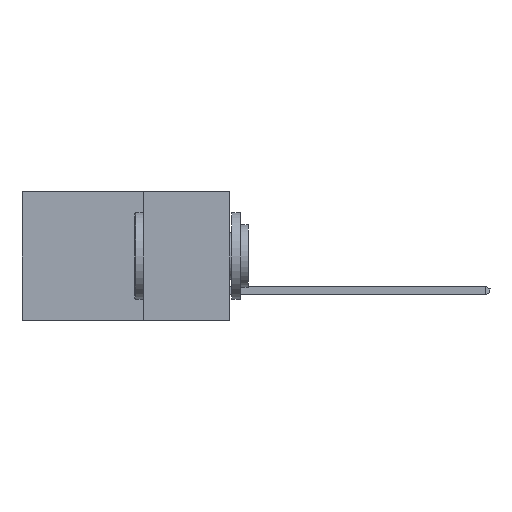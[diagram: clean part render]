
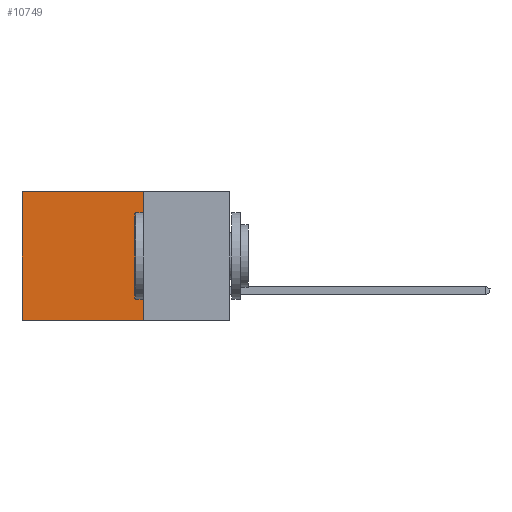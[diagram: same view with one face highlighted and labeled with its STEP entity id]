
A CAD part, left-side view. The second image highlights one B-rep face of the part: STEP entity #10749.
In plain terms, the highlighted planar face has unit normal (-1, 0, 0).
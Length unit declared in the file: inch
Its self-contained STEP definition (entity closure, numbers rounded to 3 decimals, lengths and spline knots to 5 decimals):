
#174 = ORIENTED_EDGE ( 'NONE', *, *, #14636, .F. ) ;
#426 = ORIENTED_EDGE ( 'NONE', *, *, #14293, .F. ) ;
#1193 = CARTESIAN_POINT ( 'NONE',  ( 0.2615, 0.25, -0.37 ) ) ;
#1228 = LINE ( 'NONE', #2352, #8386 ) ;
#1419 = CARTESIAN_POINT ( 'NONE',  ( 0.2615, 0.25, -0.37 ) ) ;
#2322 = LINE ( 'NONE', #1193, #9611 ) ;
#2352 = CARTESIAN_POINT ( 'NONE',  ( 0.2615, 0.6, -0.37 ) ) ;
#2372 = DIRECTION ( 'NONE',  ( 1., 0., 0. ) ) ;
#2518 = FACE_OUTER_BOUND ( 'NONE', #10405, .T. ) ;
#2593 = CARTESIAN_POINT ( 'NONE',  ( 0.2615, 0.25, 0. ) ) ;
#3091 = VERTEX_POINT ( 'NONE', #1419 ) ;
#3502 = PLANE ( 'NONE',  #11160 ) ;
#3981 = ORIENTED_EDGE ( 'NONE', *, *, #9873, .T. ) ;
#4097 = VERTEX_POINT ( 'NONE', #6072 ) ;
#4595 = CARTESIAN_POINT ( 'NONE',  ( 0.2615, 0.6, -0.37 ) ) ;
#5292 = LINE ( 'NONE', #7529, #10825 ) ;
#5918 = CARTESIAN_POINT ( 'NONE',  ( 0.2615, 0.25, 0. ) ) ;
#6072 = CARTESIAN_POINT ( 'NONE',  ( 0.2615, 0.6, 0. ) ) ;
#6815 = DIRECTION ( 'NONE',  ( 0., 1., 0. ) ) ;
#7054 = VERTEX_POINT ( 'NONE', #4595 ) ;
#7094 = CARTESIAN_POINT ( 'NONE',  ( 0.2615, 0.25, -0.37 ) ) ;
#7529 = CARTESIAN_POINT ( 'NONE',  ( 0.2615, 0.25, -0.37 ) ) ;
#8386 = VECTOR ( 'NONE', #8938, 39.37008 ) ;
#8902 = VECTOR ( 'NONE', #10819, 39.37008 ) ;
#8938 = DIRECTION ( 'NONE',  ( 0., 0., -1. ) ) ;
#9409 = ORIENTED_EDGE ( 'NONE', *, *, #14449, .T. ) ;
#9477 = LINE ( 'NONE', #2593, #8902 ) ;
#9611 = VECTOR ( 'NONE', #6815, 39.37008 ) ;
#9873 = EDGE_CURVE ( 'NONE', #4097, #7054, #1228, .T. ) ;
#10314 = VERTEX_POINT ( 'NONE', #5918 ) ;
#10405 = EDGE_LOOP ( 'NONE', ( #3981, #426, #174, #9409 ) ) ;
#10749 = ADVANCED_FACE ( 'NONE', ( #2518 ), #3502, .F. ) ;
#10819 = DIRECTION ( 'NONE',  ( 0., 1., 0. ) ) ;
#10825 = VECTOR ( 'NONE', #11188, 39.37008 ) ;
#11160 = AXIS2_PLACEMENT_3D ( 'NONE', #7094, #2372, #11578 ) ;
#11188 = DIRECTION ( 'NONE',  ( 0., 0., -1. ) ) ;
#11578 = DIRECTION ( 'NONE',  ( 0., 0., -1. ) ) ;
#14293 = EDGE_CURVE ( 'NONE', #3091, #7054, #2322, .T. ) ;
#14449 = EDGE_CURVE ( 'NONE', #10314, #4097, #9477, .T. ) ;
#14636 = EDGE_CURVE ( 'NONE', #10314, #3091, #5292, .T. ) ;
